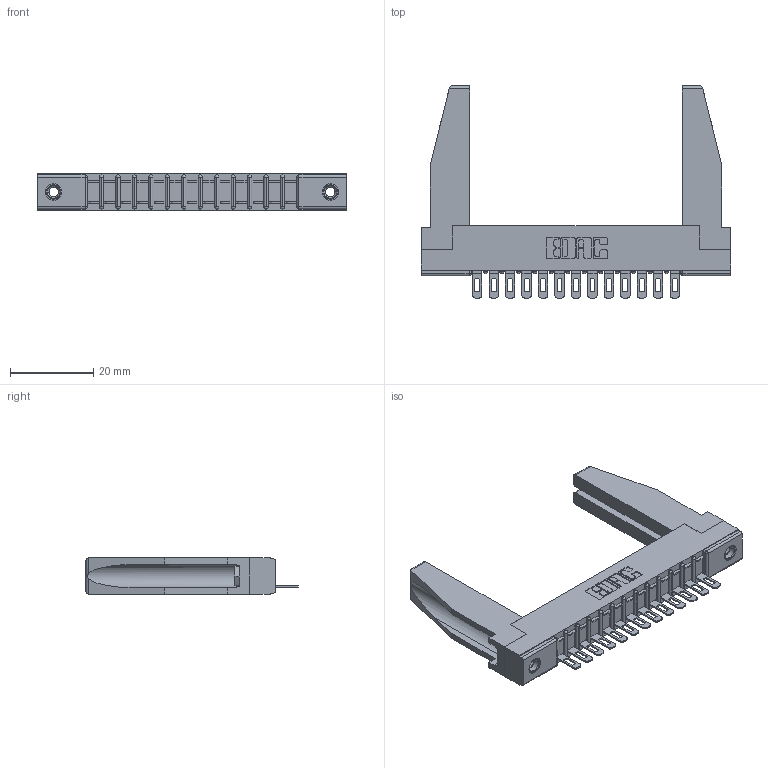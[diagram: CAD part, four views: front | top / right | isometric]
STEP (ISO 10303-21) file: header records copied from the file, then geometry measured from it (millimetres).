
FILE_DESCRIPTION (( 'STEP AP203' ), '1' );
FILE_NAME ('357-013-501-178.STEP', '2019-09-16T19:28:40', ( '' ), ( '' ), 'SwSTEP 2.0', 'SolidWorks 2016', '' );
FILE_SCHEMA (( 'CONFIG_CONTROL_DESIGN' ));
Length unit declared in the file: inch
Products named in the file (5): 345-250-001_345-250-001-102; 307-290-002_501; 307-220-078; 307 Part_.156 Dia Mounting Holes; 357-013-501-178
Assembly tree (18 placements, depth 2):
  357-013-501-178
    307 Part_.156 Dia Mounting Holes
    307-290-002_501  x13
    307-220-078  x2
    345-250-001_345-250-001-102  x2
Bounding box: 74.52 x 51.13 x 8.71 mm (x, y, z)
Volume: 8919.8 mm3; surface area: 12368.4 mm2
Topology: 18 solids, 18 shells, 1250 faces, 3747 edges, 2450 vertices
Faces by surface type: plane 726, cylinder 480, sphere 28, cone 12, torus 4
Entity records: 17953 total; most frequent: CARTESIAN_POINT 3022, ORIENTED_EDGE 2968, DIRECTION 2910, EDGE_CURVE 1484, VECTOR 1122, LINE 1122, VERTEX_POINT 964, AXIS2_PLACEMENT_3D 894
